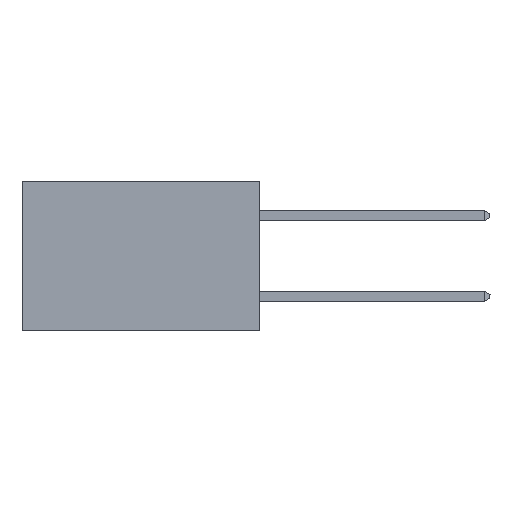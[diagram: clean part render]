
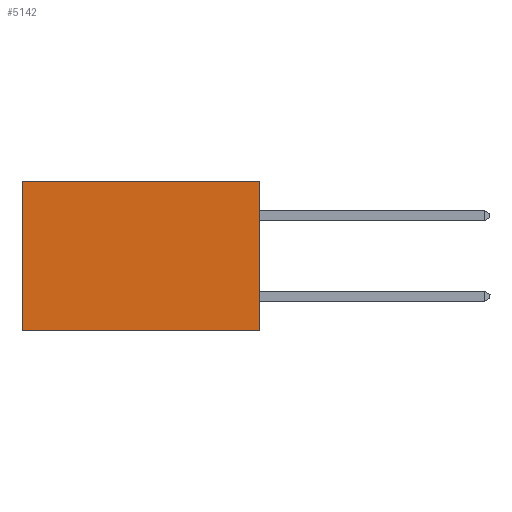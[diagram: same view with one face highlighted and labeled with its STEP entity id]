
A CAD part, left-side view. The second image highlights one B-rep face of the part: STEP entity #5142.
In plain terms, the highlighted planar face has unit normal (-1, 0, 0).
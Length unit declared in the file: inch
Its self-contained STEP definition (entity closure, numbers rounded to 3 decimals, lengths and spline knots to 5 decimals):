
#8 = EDGE_CURVE ( 'NONE', #5320, #3538, #2545, .T. ) ;
#756 = CARTESIAN_POINT ( 'NONE',  ( 0.277, 0., -0.37 ) ) ;
#910 = VECTOR ( 'NONE', #4738, 39.37008 ) ;
#1185 = LINE ( 'NONE', #4848, #910 ) ;
#1332 = CARTESIAN_POINT ( 'NONE',  ( 0.277, 0., 0. ) ) ;
#1584 = EDGE_CURVE ( 'NONE', #3538, #5006, #6665, .T. ) ;
#1846 = VERTEX_POINT ( 'NONE', #6782 ) ;
#1935 = ORIENTED_EDGE ( 'NONE', *, *, #5185, .T. ) ;
#2010 = VECTOR ( 'NONE', #5556, 39.37008 ) ;
#2322 = VECTOR ( 'NONE', #7358, 39.37008 ) ;
#2446 = ORIENTED_EDGE ( 'NONE', *, *, #2700, .T. ) ;
#2545 = LINE ( 'NONE', #5868, #2322 ) ;
#2694 = DIRECTION ( 'NONE',  ( 1., 0., 0. ) ) ;
#2700 = EDGE_CURVE ( 'NONE', #1846, #5006, #1185, .T. ) ;
#2856 = ORIENTED_EDGE ( 'NONE', *, *, #1584, .F. ) ;
#3259 = ORIENTED_EDGE ( 'NONE', *, *, #8, .F. ) ;
#3538 = VERTEX_POINT ( 'NONE', #6958 ) ;
#4506 = CARTESIAN_POINT ( 'NONE',  ( 0.277, 0., -0.37 ) ) ;
#4738 = DIRECTION ( 'NONE',  ( 0., 0., -1. ) ) ;
#4848 = CARTESIAN_POINT ( 'NONE',  ( 0.277, 0.59, -0.37 ) ) ;
#5006 = VERTEX_POINT ( 'NONE', #7413 ) ;
#5111 = EDGE_LOOP ( 'NONE', ( #2446, #2856, #3259, #1935 ) ) ;
#5142 = ADVANCED_FACE ( 'NONE', ( #5306 ), #7432, .F. ) ;
#5143 = VECTOR ( 'NONE', #6089, 39.37008 ) ;
#5185 = EDGE_CURVE ( 'NONE', #5320, #1846, #7610, .T. ) ;
#5306 = FACE_OUTER_BOUND ( 'NONE', #5111, .T. ) ;
#5320 = VERTEX_POINT ( 'NONE', #6110 ) ;
#5556 = DIRECTION ( 'NONE',  ( 0., 1., 0. ) ) ;
#5868 = CARTESIAN_POINT ( 'NONE',  ( 0.277, 0., -0.37 ) ) ;
#6074 = AXIS2_PLACEMENT_3D ( 'NONE', #4506, #2694, #6552 ) ;
#6089 = DIRECTION ( 'NONE',  ( 0., 1., 0. ) ) ;
#6110 = CARTESIAN_POINT ( 'NONE',  ( 0.277, 0., 0. ) ) ;
#6552 = DIRECTION ( 'NONE',  ( 0., 0., -1. ) ) ;
#6665 = LINE ( 'NONE', #756, #2010 ) ;
#6782 = CARTESIAN_POINT ( 'NONE',  ( 0.277, 0.59, 0. ) ) ;
#6958 = CARTESIAN_POINT ( 'NONE',  ( 0.277, 0., -0.37 ) ) ;
#7358 = DIRECTION ( 'NONE',  ( 0., 0., -1. ) ) ;
#7413 = CARTESIAN_POINT ( 'NONE',  ( 0.277, 0.59, -0.37 ) ) ;
#7432 = PLANE ( 'NONE',  #6074 ) ;
#7610 = LINE ( 'NONE', #1332, #5143 ) ;
